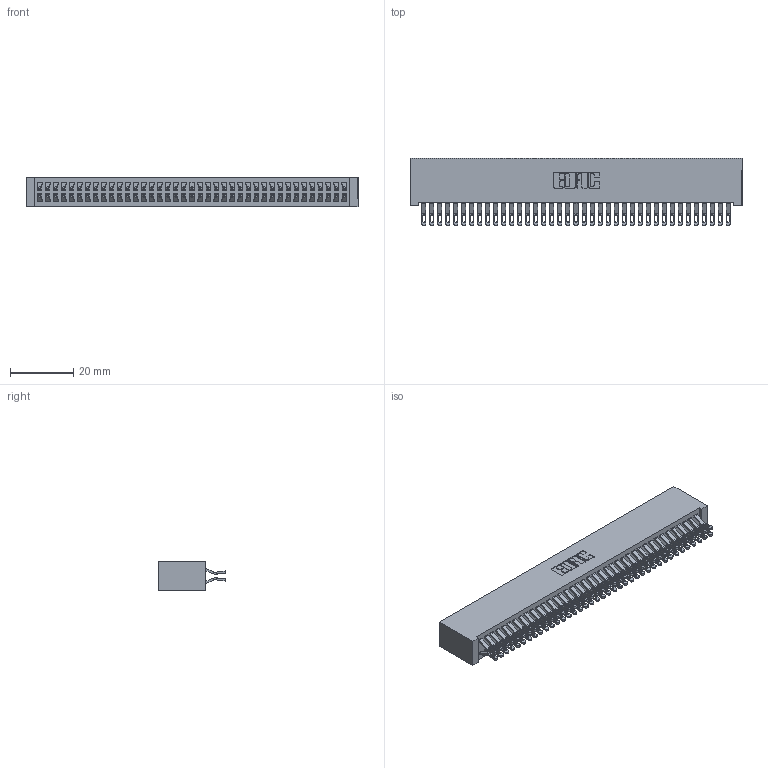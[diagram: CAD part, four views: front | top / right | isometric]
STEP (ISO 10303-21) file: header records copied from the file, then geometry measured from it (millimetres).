
FILE_DESCRIPTION (( 'STEP AP203' ), '1' );
FILE_NAME ('392-078-555-201.STEP', '2019-10-09T14:07:33', ( '' ), ( '' ), 'SwSTEP 2.0', 'SolidWorks 2016', '' );
FILE_SCHEMA (( 'CONFIG_CONTROL_DESIGN' ));
Length unit declared in the file: inch
Products named in the file (3): 342 Part_Lugless; 345-292-001_555 Tail; 392-078-555-201
Assembly tree (79 placements, depth 2):
  392-078-555-201
    342 Part_Lugless
    345-292-001_555 Tail  x78
Bounding box: 105.31 x 21.47 x 9.4 mm (x, y, z)
Volume: 10104 mm3; surface area: 17573.8 mm2
Topology: 79 solids, 79 shells, 4626 faces, 14549 edges, 9698 vertices
Faces by surface type: plane 2714, cylinder 1912
Entity records: 25395 total; most frequent: CARTESIAN_POINT 4244, ORIENTED_EDGE 4150, DIRECTION 3595, EDGE_CURVE 2075, LINE 1935, VECTOR 1935, VERTEX_POINT 1382, AXIS2_PLACEMENT_3D 830
